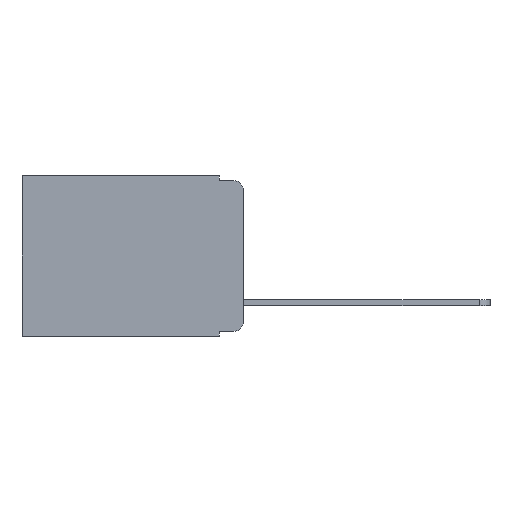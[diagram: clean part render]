
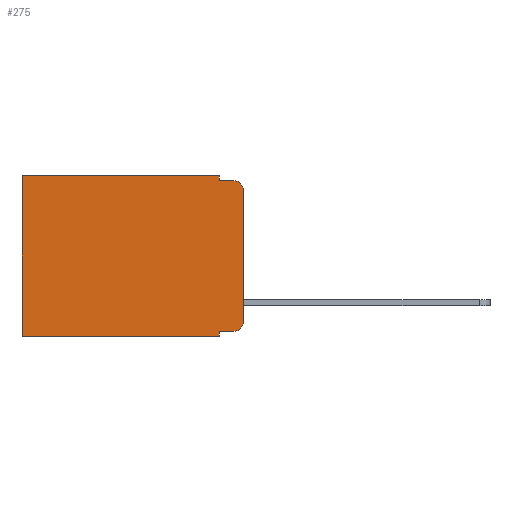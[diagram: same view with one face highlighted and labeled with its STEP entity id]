
A CAD part, left-side view. The second image highlights one B-rep face of the part: STEP entity #275.
In plain terms, the highlighted planar face has unit normal (-1, 0, 0).
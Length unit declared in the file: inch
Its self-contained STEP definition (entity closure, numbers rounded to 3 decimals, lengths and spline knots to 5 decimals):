
#14 = ORIENTED_EDGE ( 'NONE', *, *, #9413, .T. ) ;
#28 = DIRECTION ( 'NONE',  ( 0., 0., -1. ) ) ;
#55 = ORIENTED_EDGE ( 'NONE', *, *, #9564, .T. ) ;
#205 = ORIENTED_EDGE ( 'NONE', *, *, #755, .F. ) ;
#275 = ADVANCED_FACE ( 'NONE', ( #3123 ), #9903, .F. ) ;
#277 = ORIENTED_EDGE ( 'NONE', *, *, #5406, .F. ) ;
#353 = CARTESIAN_POINT ( 'NONE',  ( 0.298, 0.051, -0.01 ) ) ;
#676 = ORIENTED_EDGE ( 'NONE', *, *, #11424, .T. ) ;
#732 = ORIENTED_EDGE ( 'NONE', *, *, #6168, .T. ) ;
#755 = EDGE_CURVE ( 'NONE', #4784, #4034, #6440, .T. ) ;
#869 = VECTOR ( 'NONE', #7079, 39.37008 ) ;
#1032 = LINE ( 'NONE', #10884, #10201 ) ;
#1101 = AXIS2_PLACEMENT_3D ( 'NONE', #10408, #10379, #2514 ) ;
#1157 = VERTEX_POINT ( 'NONE', #4145 ) ;
#1421 = AXIS2_PLACEMENT_3D ( 'NONE', #9851, #11206, #11221 ) ;
#1429 = CARTESIAN_POINT ( 'NONE',  ( 0.298, 0., 0. ) ) ;
#1506 = EDGE_LOOP ( 'NONE', ( #2671, #3780, #4333, #4541, #14, #55, #205, #277, #676, #732 ) ) ;
#1571 = LINE ( 'NONE', #1429, #869 ) ;
#1656 = VERTEX_POINT ( 'NONE', #2075 ) ;
#1849 = CARTESIAN_POINT ( 'NONE',  ( 0.298, 0.051, 0. ) ) ;
#2041 = VERTEX_POINT ( 'NONE', #11232 ) ;
#2075 = CARTESIAN_POINT ( 'NONE',  ( 0.298, 0.051, 0. ) ) ;
#2130 = EDGE_CURVE ( 'NONE', #6848, #11375, #1571, .T. ) ;
#2224 = CARTESIAN_POINT ( 'NONE',  ( 0.298, 0.051, -0.333 ) ) ;
#2424 = LINE ( 'NONE', #7707, #11679 ) ;
#2514 = DIRECTION ( 'NONE',  ( 0., 0., -1. ) ) ;
#2671 = ORIENTED_EDGE ( 'NONE', *, *, #2130, .F. ) ;
#2807 = DIRECTION ( 'NONE',  ( 0., 0., -1. ) ) ;
#2862 = VECTOR ( 'NONE', #28, 39.37008 ) ;
#3123 = FACE_OUTER_BOUND ( 'NONE', #1506, .T. ) ;
#3124 = CIRCLE ( 'NONE', #9211, 0.02 ) ;
#3407 = EDGE_CURVE ( 'NONE', #6848, #2041, #9931, .T. ) ;
#3780 = ORIENTED_EDGE ( 'NONE', *, *, #3407, .T. ) ;
#4019 = EDGE_CURVE ( 'NONE', #6208, #2041, #6356, .T. ) ;
#4034 = VERTEX_POINT ( 'NONE', #9870 ) ;
#4145 = CARTESIAN_POINT ( 'NONE',  ( 0.298, 0.473, 0. ) ) ;
#4269 = CARTESIAN_POINT ( 'NONE',  ( 0.298, 0.051, 0. ) ) ;
#4333 = ORIENTED_EDGE ( 'NONE', *, *, #4019, .F. ) ;
#4541 = ORIENTED_EDGE ( 'NONE', *, *, #5833, .F. ) ;
#4657 = DIRECTION ( 'NONE',  ( 0., 1., 0. ) ) ;
#4673 = CARTESIAN_POINT ( 'NONE',  ( 0.298, 0.051, -0.343 ) ) ;
#4784 = VERTEX_POINT ( 'NONE', #4673 ) ;
#4810 = CARTESIAN_POINT ( 'NONE',  ( 0.298, 0.02, -0.333 ) ) ;
#4872 = VERTEX_POINT ( 'NONE', #4810 ) ;
#5262 = DIRECTION ( 'NONE',  ( -1., 0., 0. ) ) ;
#5406 = EDGE_CURVE ( 'NONE', #12039, #4784, #9753, .T. ) ;
#5685 = CARTESIAN_POINT ( 'NONE',  ( 0.298, 0., -0.343 ) ) ;
#5833 = EDGE_CURVE ( 'NONE', #1656, #6208, #8021, .T. ) ;
#6168 = EDGE_CURVE ( 'NONE', #4872, #11375, #3124, .T. ) ;
#6208 = VERTEX_POINT ( 'NONE', #353 ) ;
#6356 = LINE ( 'NONE', #8374, #10182 ) ;
#6440 = LINE ( 'NONE', #5685, #10542 ) ;
#6848 = VERTEX_POINT ( 'NONE', #7670 ) ;
#7074 = VECTOR ( 'NONE', #7570, 39.37008 ) ;
#7079 = DIRECTION ( 'NONE',  ( 0., 0., -1. ) ) ;
#7570 = DIRECTION ( 'NONE',  ( 0., 0., -1. ) ) ;
#7670 = CARTESIAN_POINT ( 'NONE',  ( 0.298, 0., -0.03 ) ) ;
#7707 = CARTESIAN_POINT ( 'NONE',  ( 0.298, 0.051, -0.333 ) ) ;
#7715 = VECTOR ( 'NONE', #2807, 39.37008 ) ;
#8021 = LINE ( 'NONE', #1849, #7715 ) ;
#8374 = CARTESIAN_POINT ( 'NONE',  ( 0.298, 0.051, -0.01 ) ) ;
#8580 = DIRECTION ( 'NONE',  ( 0., -1., 0. ) ) ;
#8915 = DIRECTION ( 'NONE',  ( 0., 1., 0. ) ) ;
#9211 = AXIS2_PLACEMENT_3D ( 'NONE', #10546, #5262, #11435 ) ;
#9413 = EDGE_CURVE ( 'NONE', #1656, #1157, #1032, .T. ) ;
#9564 = EDGE_CURVE ( 'NONE', #1157, #4034, #11709, .T. ) ;
#9753 = LINE ( 'NONE', #4269, #2862 ) ;
#9851 = CARTESIAN_POINT ( 'NONE',  ( 0.298, 0., 0. ) ) ;
#9870 = CARTESIAN_POINT ( 'NONE',  ( 0.298, 0.473, -0.343 ) ) ;
#9903 = PLANE ( 'NONE',  #1421 ) ;
#9931 = CIRCLE ( 'NONE', #1101, 0.02 ) ;
#10180 = DIRECTION ( 'NONE',  ( 0., -1., 0. ) ) ;
#10182 = VECTOR ( 'NONE', #10180, 39.37008 ) ;
#10201 = VECTOR ( 'NONE', #4657, 39.37008 ) ;
#10379 = DIRECTION ( 'NONE',  ( -1., 0., 0. ) ) ;
#10408 = CARTESIAN_POINT ( 'NONE',  ( 0.298, 0.02, -0.03 ) ) ;
#10542 = VECTOR ( 'NONE', #8915, 39.37008 ) ;
#10546 = CARTESIAN_POINT ( 'NONE',  ( 0.298, 0.02, -0.313 ) ) ;
#10884 = CARTESIAN_POINT ( 'NONE',  ( 0.298, 0., 0. ) ) ;
#11132 = CARTESIAN_POINT ( 'NONE',  ( 0.298, 0., -0.313 ) ) ;
#11206 = DIRECTION ( 'NONE',  ( 1., 0., 0. ) ) ;
#11221 = DIRECTION ( 'NONE',  ( 0., 0., -1. ) ) ;
#11232 = CARTESIAN_POINT ( 'NONE',  ( 0.298, 0.02, -0.01 ) ) ;
#11375 = VERTEX_POINT ( 'NONE', #11132 ) ;
#11424 = EDGE_CURVE ( 'NONE', #12039, #4872, #2424, .T. ) ;
#11435 = DIRECTION ( 'NONE',  ( 0., 0., -1. ) ) ;
#11679 = VECTOR ( 'NONE', #8580, 39.37008 ) ;
#11709 = LINE ( 'NONE', #11879, #7074 ) ;
#11879 = CARTESIAN_POINT ( 'NONE',  ( 0.298, 0.473, 0. ) ) ;
#12039 = VERTEX_POINT ( 'NONE', #2224 ) ;
